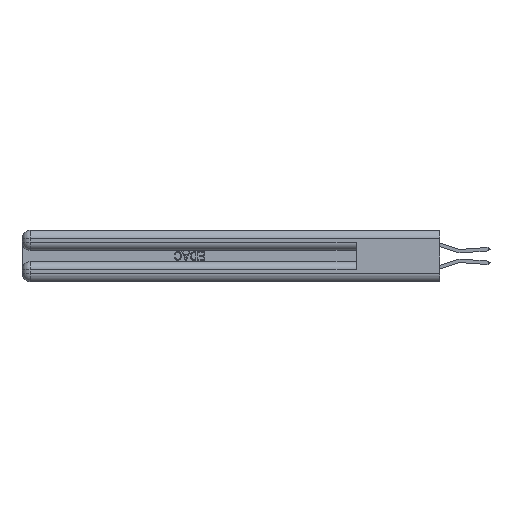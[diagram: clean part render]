
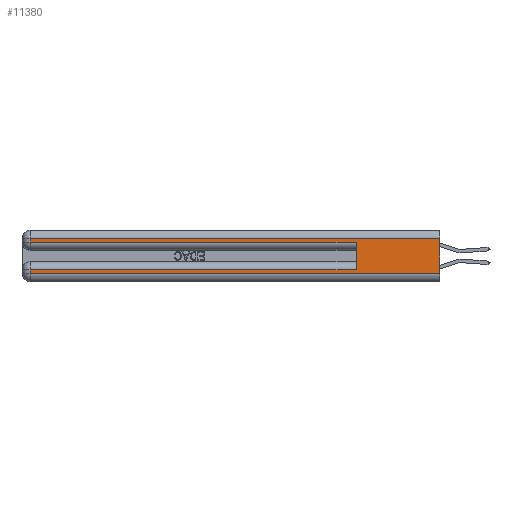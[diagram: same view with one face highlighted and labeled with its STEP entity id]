
A CAD part, left-side view. The second image highlights one B-rep face of the part: STEP entity #11380.
In plain terms, the highlighted planar face has unit normal (-1, 0, 0).
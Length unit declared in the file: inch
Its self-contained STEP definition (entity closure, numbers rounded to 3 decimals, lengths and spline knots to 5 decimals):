
#623 = VERTEX_POINT ( 'NONE', #26256 ) ;
#2229 = DIRECTION ( 'NONE',  ( 0., -1., 0. ) ) ;
#3004 = FACE_OUTER_BOUND ( 'NONE', #19384, .T. ) ;
#3684 = ORIENTED_EDGE ( 'NONE', *, *, #15642, .T. ) ;
#3700 = VECTOR ( 'NONE', #21581, 39.37008 ) ;
#3943 = ORIENTED_EDGE ( 'NONE', *, *, #42527, .T. ) ;
#4184 = DIRECTION ( 'NONE',  ( 0., 0., -1. ) ) ;
#4213 = VERTEX_POINT ( 'NONE', #7426 ) ;
#4442 = CARTESIAN_POINT ( 'NONE',  ( 0., 0., 0.37 ) ) ;
#4482 = DIRECTION ( 'NONE',  ( 0., 0., 1. ) ) ;
#5299 = DIRECTION ( 'NONE',  ( 0., 1., 0. ) ) ;
#5776 = LINE ( 'NONE', #24004, #30877 ) ;
#7062 = CARTESIAN_POINT ( 'NONE',  ( 0., 2.94, 0.37 ) ) ;
#7426 = CARTESIAN_POINT ( 'NONE',  ( 0., 2.94, 0.085 ) ) ;
#8331 = VECTOR ( 'NONE', #39593, 39.37008 ) ;
#8559 = ORIENTED_EDGE ( 'NONE', *, *, #45845, .T. ) ;
#8719 = LINE ( 'NONE', #36462, #29297 ) ;
#10338 = VERTEX_POINT ( 'NONE', #30267 ) ;
#11155 = ORIENTED_EDGE ( 'NONE', *, *, #35579, .T. ) ;
#11344 = CARTESIAN_POINT ( 'NONE',  ( 0., 0.6, 0.145 ) ) ;
#11380 = ADVANCED_FACE ( 'NONE', ( #3004 ), #46605, .F. ) ;
#12053 = VECTOR ( 'NONE', #4482, 39.37008 ) ;
#12609 = LINE ( 'NONE', #11344, #12053 ) ;
#13863 = CARTESIAN_POINT ( 'NONE',  ( 0., 0., 0.06 ) ) ;
#14402 = CARTESIAN_POINT ( 'NONE',  ( 0., 0.6, 0.085 ) ) ;
#15160 = VECTOR ( 'NONE', #5299, 39.37008 ) ;
#15642 = EDGE_CURVE ( 'NONE', #27355, #40058, #40174, .T. ) ;
#17884 = VECTOR ( 'NONE', #23446, 39.37008 ) ;
#19384 = EDGE_LOOP ( 'NONE', ( #22700, #38526, #21400, #8559, #42860, #11155, #3943, #3684 ) ) ;
#20197 = VECTOR ( 'NONE', #28269, 39.37008 ) ;
#20566 = DIRECTION ( 'NONE',  ( 1., 0., 0. ) ) ;
#21400 = ORIENTED_EDGE ( 'NONE', *, *, #28138, .T. ) ;
#21581 = DIRECTION ( 'NONE',  ( 0., 0., -1. ) ) ;
#21971 = DIRECTION ( 'NONE',  ( 0., 1., 0. ) ) ;
#22082 = LINE ( 'NONE', #34812, #15160 ) ;
#22700 = ORIENTED_EDGE ( 'NONE', *, *, #30532, .F. ) ;
#22752 = VERTEX_POINT ( 'NONE', #14402 ) ;
#23446 = DIRECTION ( 'NONE',  ( 0., 0., -1. ) ) ;
#24004 = CARTESIAN_POINT ( 'NONE',  ( 0., 0., 0.285 ) ) ;
#26256 = CARTESIAN_POINT ( 'NONE',  ( 0., 0.6, 0.285 ) ) ;
#26423 = LINE ( 'NONE', #30460, #17884 ) ;
#27007 = CARTESIAN_POINT ( 'NONE',  ( 0., 2.94, 0.06 ) ) ;
#27268 = EDGE_CURVE ( 'NONE', #10338, #41853, #22082, .T. ) ;
#27355 = VERTEX_POINT ( 'NONE', #27007 ) ;
#28046 = CARTESIAN_POINT ( 'NONE',  ( 0., 2.94, 0.31 ) ) ;
#28138 = EDGE_CURVE ( 'NONE', #41853, #41446, #35739, .T. ) ;
#28269 = DIRECTION ( 'NONE',  ( 0., -1., 0. ) ) ;
#28683 = CARTESIAN_POINT ( 'NONE',  ( 0., 2.94, 0.37 ) ) ;
#28902 = LINE ( 'NONE', #7062, #3700 ) ;
#29297 = VECTOR ( 'NONE', #21971, 39.37008 ) ;
#30267 = CARTESIAN_POINT ( 'NONE',  ( 0., 0., 0.31 ) ) ;
#30460 = CARTESIAN_POINT ( 'NONE',  ( 0., 0., 0.37 ) ) ;
#30532 = EDGE_CURVE ( 'NONE', #10338, #40058, #26423, .T. ) ;
#30877 = VECTOR ( 'NONE', #2229, 39.37008 ) ;
#32553 = CARTESIAN_POINT ( 'NONE',  ( 0., 0., 0.06 ) ) ;
#33893 = CARTESIAN_POINT ( 'NONE',  ( 0., 2.94, 0.285 ) ) ;
#33984 = AXIS2_PLACEMENT_3D ( 'NONE', #4442, #20566, #4184 ) ;
#34812 = CARTESIAN_POINT ( 'NONE',  ( 0., 0., 0.31 ) ) ;
#35579 = EDGE_CURVE ( 'NONE', #22752, #4213, #8719, .T. ) ;
#35739 = LINE ( 'NONE', #28683, #8331 ) ;
#36462 = CARTESIAN_POINT ( 'NONE',  ( 0., 0., 0.085 ) ) ;
#38526 = ORIENTED_EDGE ( 'NONE', *, *, #27268, .T. ) ;
#39593 = DIRECTION ( 'NONE',  ( 0., 0., -1. ) ) ;
#40058 = VERTEX_POINT ( 'NONE', #32553 ) ;
#40174 = LINE ( 'NONE', #13863, #20197 ) ;
#41446 = VERTEX_POINT ( 'NONE', #33893 ) ;
#41853 = VERTEX_POINT ( 'NONE', #28046 ) ;
#42527 = EDGE_CURVE ( 'NONE', #4213, #27355, #28902, .T. ) ;
#42860 = ORIENTED_EDGE ( 'NONE', *, *, #45611, .F. ) ;
#45611 = EDGE_CURVE ( 'NONE', #22752, #623, #12609, .T. ) ;
#45845 = EDGE_CURVE ( 'NONE', #41446, #623, #5776, .T. ) ;
#46605 = PLANE ( 'NONE',  #33984 ) ;
